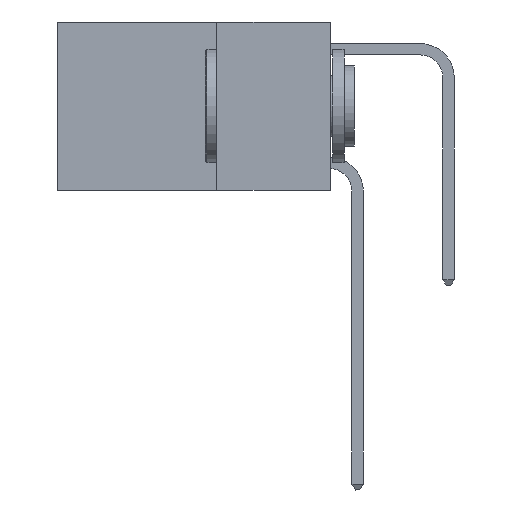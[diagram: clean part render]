
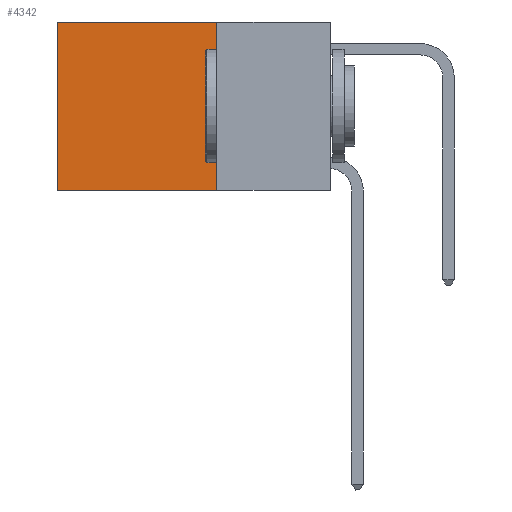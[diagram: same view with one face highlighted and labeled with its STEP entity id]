
A CAD part, left-side view. The second image highlights one B-rep face of the part: STEP entity #4342.
In plain terms, the highlighted planar face has unit normal (-1, 0, 0).
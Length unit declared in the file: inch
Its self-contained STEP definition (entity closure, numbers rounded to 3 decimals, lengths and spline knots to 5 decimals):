
#323 = VECTOR ( 'NONE', #13643, 39.37008 ) ;
#843 = FACE_OUTER_BOUND ( 'NONE', #16597, .T. ) ;
#1026 = LINE ( 'NONE', #18062, #323 ) ;
#1559 = VECTOR ( 'NONE', #7829, 39.37008 ) ;
#1932 = CARTESIAN_POINT ( 'NONE',  ( 0.2625, 0.6, -0.37 ) ) ;
#2692 = EDGE_CURVE ( 'NONE', #8386, #14307, #6133, .T. ) ;
#2725 = CARTESIAN_POINT ( 'NONE',  ( 0.2625, 0.25, 0. ) ) ;
#4342 = ADVANCED_FACE ( 'NONE', ( #843 ), #8771, .F. ) ;
#4735 = CARTESIAN_POINT ( 'NONE',  ( 0.2625, 0.25, -0.37 ) ) ;
#5100 = EDGE_CURVE ( 'NONE', #14307, #12700, #17971, .T. ) ;
#6133 = LINE ( 'NONE', #2725, #17322 ) ;
#6957 = CARTESIAN_POINT ( 'NONE',  ( 0.2625, 0.25, 0. ) ) ;
#7775 = LINE ( 'NONE', #6957, #12303 ) ;
#7829 = DIRECTION ( 'NONE',  ( 0., 0., -1. ) ) ;
#8386 = VERTEX_POINT ( 'NONE', #15213 ) ;
#8771 = PLANE ( 'NONE',  #18876 ) ;
#10220 = ORIENTED_EDGE ( 'NONE', *, *, #5100, .T. ) ;
#11026 = DIRECTION ( 'NONE',  ( 1., 0., 0. ) ) ;
#12303 = VECTOR ( 'NONE', #20372, 39.37008 ) ;
#12700 = VERTEX_POINT ( 'NONE', #1932 ) ;
#12735 = ORIENTED_EDGE ( 'NONE', *, *, #17646, .F. ) ;
#13643 = DIRECTION ( 'NONE',  ( 0., 1., 0. ) ) ;
#14267 = VERTEX_POINT ( 'NONE', #4735 ) ;
#14307 = VERTEX_POINT ( 'NONE', #18239 ) ;
#15213 = CARTESIAN_POINT ( 'NONE',  ( 0.2625, 0.25, 0. ) ) ;
#16597 = EDGE_LOOP ( 'NONE', ( #10220, #22011, #12735, #23051 ) ) ;
#17322 = VECTOR ( 'NONE', #18355, 39.37008 ) ;
#17646 = EDGE_CURVE ( 'NONE', #8386, #14267, #7775, .T. ) ;
#17971 = LINE ( 'NONE', #18967, #1559 ) ;
#18062 = CARTESIAN_POINT ( 'NONE',  ( 0.2625, 0.25, -0.37 ) ) ;
#18239 = CARTESIAN_POINT ( 'NONE',  ( 0.2625, 0.6, 0. ) ) ;
#18355 = DIRECTION ( 'NONE',  ( 0., 1., 0. ) ) ;
#18876 = AXIS2_PLACEMENT_3D ( 'NONE', #24421, #11026, #26652 ) ;
#18967 = CARTESIAN_POINT ( 'NONE',  ( 0.2625, 0.6, 0. ) ) ;
#20269 = EDGE_CURVE ( 'NONE', #14267, #12700, #1026, .T. ) ;
#20372 = DIRECTION ( 'NONE',  ( 0., 0., -1. ) ) ;
#22011 = ORIENTED_EDGE ( 'NONE', *, *, #20269, .F. ) ;
#23051 = ORIENTED_EDGE ( 'NONE', *, *, #2692, .T. ) ;
#24421 = CARTESIAN_POINT ( 'NONE',  ( 0.2625, 0.25, 0. ) ) ;
#26652 = DIRECTION ( 'NONE',  ( 0., 0., -1. ) ) ;
